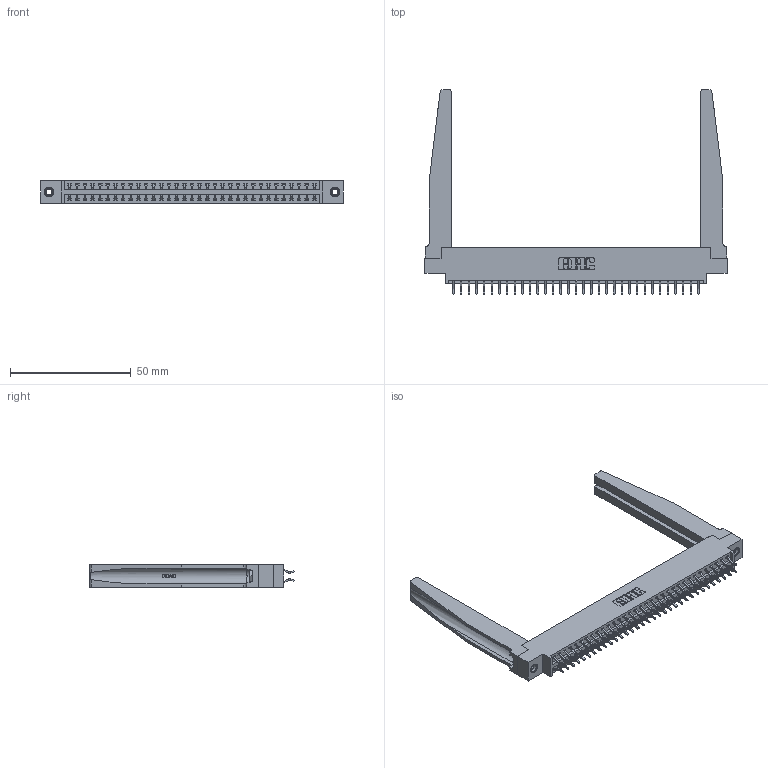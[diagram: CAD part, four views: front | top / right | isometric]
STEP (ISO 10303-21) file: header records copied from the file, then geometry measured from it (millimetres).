
FILE_DESCRIPTION (( 'STEP AP203' ), '1' );
FILE_NAME ('346-066-556-878.STEP', '2022-05-24T17:52:43', ( '' ), ( '' ), 'SwSTEP 2.0', 'SolidWorks 2020', '' );
FILE_SCHEMA (( 'CONFIG_CONTROL_DESIGN' ));
Length unit declared in the file: inch
Products named in the file (5): 346 Part_0.170 Offset - 0.156 Dia-TH; 345-250-001_345-250-001-102; 345-292-001_556 Tail; 346-220-078_345-220-078; 346-066-556-878
Assembly tree (71 placements, depth 2):
  346-066-556-878
    346 Part_0.170 Offset - 0.156 Dia-TH
    345-292-001_556 Tail  x66
    346-220-078_345-220-078  x2
    345-250-001_345-250-001-102  x2
Bounding box: 125.35 x 84.84 x 9.4 mm (x, y, z)
Volume: 18886.7 mm3; surface area: 23013.3 mm2
Topology: 71 solids, 71 shells, 4202 faces, 12403 edges, 8170 vertices
Faces by surface type: plane 2810, cylinder 1340, bspline 36, cone 12, torus 4
Entity records: 28264 total; most frequent: CARTESIAN_POINT 5629, ORIENTED_EDGE 4438, DIRECTION 3985, EDGE_CURVE 2219, LINE 1853, VECTOR 1853, VERTEX_POINT 1472, AXIS2_PLACEMENT_3D 1066
